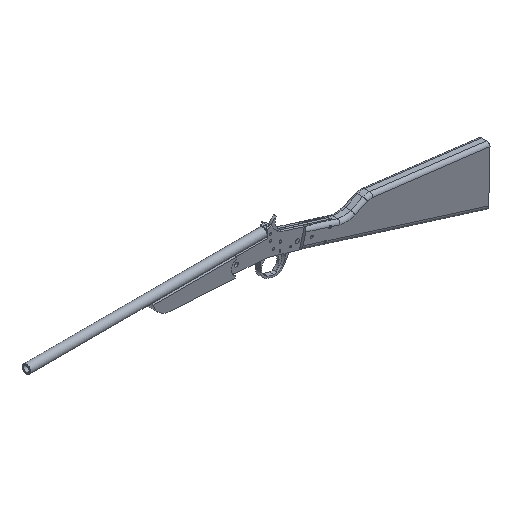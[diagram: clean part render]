
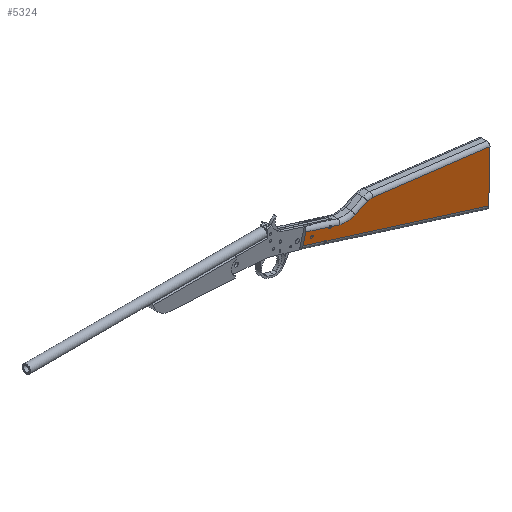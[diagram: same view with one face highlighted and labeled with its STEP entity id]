
A CAD part, isometric view. The second image highlights one B-rep face of the part: STEP entity #5324.
In plain terms, the highlighted planar face has unit normal (0, -1, 0).
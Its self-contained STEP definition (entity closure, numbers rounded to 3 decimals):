
#547=PLANE('',#6312);
#773=FACE_OUTER_BOUND('',#1126,.T.);
#1126=EDGE_LOOP('',(#4203,#4204,#4205,#4206,#4207,#4208,#4209,#4210));
#1484=LINE('',#15313,#1871);
#1501=LINE('',#15353,#1888);
#1524=LINE('',#15578,#1911);
#1526=LINE('',#15584,#1913);
#1527=LINE('',#15615,#1914);
#1528=LINE('',#15617,#1915);
#1871=VECTOR('',#7262,10.);
#1888=VECTOR('',#7295,10.);
#1911=VECTOR('',#7370,10.);
#1913=VECTOR('',#7376,10.);
#1914=VECTOR('',#7383,10.);
#1915=VECTOR('',#7386,10.);
#2226=CIRCLE('',#6305,19.936);
#2227=CIRCLE('',#6310,53.121);
#2566=VERTEX_POINT('',#15310);
#2567=VERTEX_POINT('',#15312);
#2582=VERTEX_POINT('',#15351);
#2606=VERTEX_POINT('',#15511);
#2607=VERTEX_POINT('',#15573);
#2608=VERTEX_POINT('',#15577);
#2610=VERTEX_POINT('',#15583);
#2611=VERTEX_POINT('',#15598);
#3130=EDGE_CURVE('',#2567,#2566,#1484,.T.);
#3151=EDGE_CURVE('',#2582,#2566,#1501,.T.);
#3190=EDGE_CURVE('',#2607,#2606,#2226,.T.);
#3191=EDGE_CURVE('',#2606,#2608,#1524,.T.);
#3194=EDGE_CURVE('',#2610,#2607,#1526,.T.);
#3196=EDGE_CURVE('',#2611,#2610,#2227,.T.);
#3198=EDGE_CURVE('',#2567,#2611,#1527,.T.);
#3199=EDGE_CURVE('',#2582,#2608,#1528,.T.);
#4203=ORIENTED_EDGE('',*,*,#3151,.F.);
#4204=ORIENTED_EDGE('',*,*,#3199,.T.);
#4205=ORIENTED_EDGE('',*,*,#3191,.F.);
#4206=ORIENTED_EDGE('',*,*,#3190,.F.);
#4207=ORIENTED_EDGE('',*,*,#3194,.F.);
#4208=ORIENTED_EDGE('',*,*,#3196,.F.);
#4209=ORIENTED_EDGE('',*,*,#3198,.F.);
#4210=ORIENTED_EDGE('',*,*,#3130,.T.);
#5324=ADVANCED_FACE('',(#773),#547,.T.);
#6305=AXIS2_PLACEMENT_3D('',#15575,#7366,#7367);
#6310=AXIS2_PLACEMENT_3D('',#15599,#7379,#7380);
#6312=AXIS2_PLACEMENT_3D('',#15616,#7384,#7385);
#7262=DIRECTION('',(-0.125,0.,-0.992));
#7295=DIRECTION('',(-0.988,0.,0.154));
#7366=DIRECTION('center_axis',(0.,1.,0.));
#7367=DIRECTION('ref_axis',(-0.299,0.,0.954));
#7370=DIRECTION('',(1.,0.,0.025));
#7376=DIRECTION('',(0.839,0.,0.544));
#7379=DIRECTION('center_axis',(0.,-1.,0.));
#7380=DIRECTION('ref_axis',(0.197,0.,-0.98));
#7383=DIRECTION('',(0.988,0.,-0.154));
#7384=DIRECTION('center_axis',(0.,-1.,0.));
#7385=DIRECTION('ref_axis',(0.,0.,
-1.));
#7386=DIRECTION('',(-0.124,0.,0.992));
#15310=CARTESIAN_POINT('',(381.828,-34.901,-328.155));
#15312=CARTESIAN_POINT('',(384.706,-34.901,-305.226));
#15313=CARTESIAN_POINT('',(385.578,-34.901,-298.278));
#15351=CARTESIAN_POINT('',(787.19,-34.901,-391.146));
#15353=CARTESIAN_POINT('',(685.59,-34.901,-375.358));
#15511=CARTESIAN_POINT('',(524.663,-34.901,-291.561));
#15573=CARTESIAN_POINT('',(514.481,-34.901,-294.753));
#15575=CARTESIAN_POINT('Origin',(525.318,-34.901,-311.486));
#15577=CARTESIAN_POINT('',(773.963,-34.901,-285.243));
#15578=CARTESIAN_POINT('',(553.96,-34.901,-290.819));
#15583=CARTESIAN_POINT('',(490.577,-34.901,-310.234));
#15584=CARTESIAN_POINT('',(517.125,-34.901,-293.041));
#15598=CARTESIAN_POINT('',(458.552,-34.901,-316.701));
#15599=CARTESIAN_POINT('Origin',(464.56,-34.901,-263.921));
#15615=CARTESIAN_POINT('',(484.749,-34.901,-320.772));
#15616=CARTESIAN_POINT('Origin',(584.528,-34.901,-339.348));
#15617=CARTESIAN_POINT('',(788.35,-34.901,-400.434));
